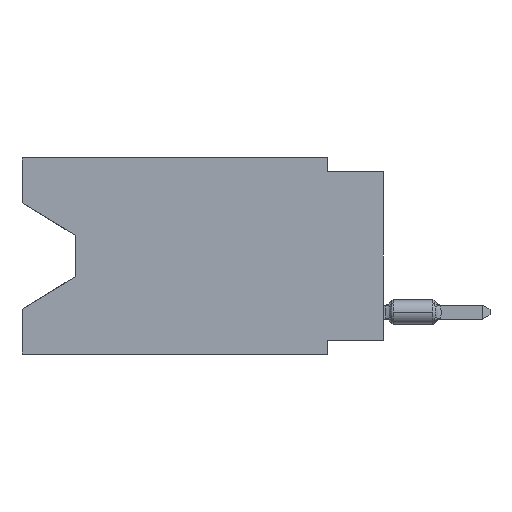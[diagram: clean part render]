
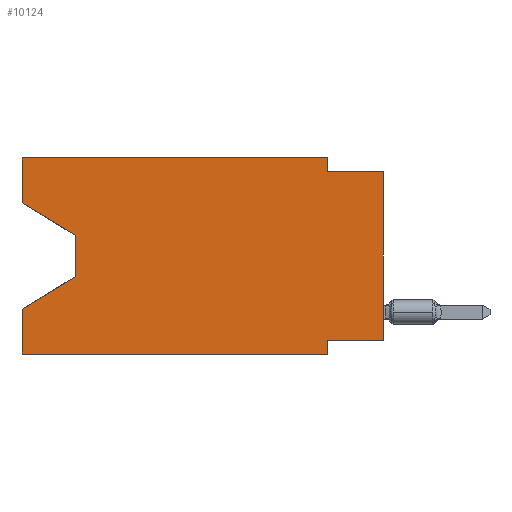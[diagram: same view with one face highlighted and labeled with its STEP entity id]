
A CAD part, left-side view. The second image highlights one B-rep face of the part: STEP entity #10124.
In plain terms, the highlighted planar face has unit normal (-1, 0, 0).
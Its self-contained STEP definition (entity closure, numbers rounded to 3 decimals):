
#159 = CARTESIAN_POINT ( 'NONE',  ( 0., 16.383, 0. ) ) ;
#282 = DIRECTION ( 'NONE',  ( 0., -0.855, -0.519 ) ) ;
#310 = VERTEX_POINT ( 'NONE', #6698 ) ;
#500 = CARTESIAN_POINT ( 'NONE',  ( 0., 2.54, -0.635 ) ) ;
#586 = ORIENTED_EDGE ( 'NONE', *, *, #6558, .F. ) ;
#632 = FACE_OUTER_BOUND ( 'NONE', #5957, .T. ) ;
#927 = VERTEX_POINT ( 'NONE', #4889 ) ;
#947 = LINE ( 'NONE', #3052, #4739 ) ;
#1186 = DIRECTION ( 'NONE',  ( 0., 0., -1. ) ) ;
#1225 = LINE ( 'NONE', #3193, #10870 ) ;
#1258 = VERTEX_POINT ( 'NONE', #9749 ) ;
#1430 = VERTEX_POINT ( 'NONE', #13397 ) ;
#1559 = ORIENTED_EDGE ( 'NONE', *, *, #10036, .F. ) ;
#1569 = VECTOR ( 'NONE', #1867, 1000. ) ;
#1867 = DIRECTION ( 'NONE',  ( 0., 0., 1. ) ) ;
#1986 = CARTESIAN_POINT ( 'NONE',  ( 0., 0., -0.635 ) ) ;
#2280 = CARTESIAN_POINT ( 'NONE',  ( 0., 13.97, -5.385 ) ) ;
#2596 = LINE ( 'NONE', #12904, #9210 ) ;
#2747 = VECTOR ( 'NONE', #8616, 1000. ) ;
#2762 = EDGE_CURVE ( 'NONE', #1430, #9212, #2888, .T. ) ;
#2861 = VECTOR ( 'NONE', #11768, 1000. ) ;
#2888 = LINE ( 'NONE', #12171, #1569 ) ;
#2956 = ORIENTED_EDGE ( 'NONE', *, *, #2762, .T. ) ;
#2991 = DIRECTION ( 'NONE',  ( 0., 0., -1. ) ) ;
#3017 = ORIENTED_EDGE ( 'NONE', *, *, #4580, .F. ) ;
#3052 = CARTESIAN_POINT ( 'NONE',  ( 0., 13.97, -5.385 ) ) ;
#3114 = VECTOR ( 'NONE', #8752, 1000. ) ;
#3193 = CARTESIAN_POINT ( 'NONE',  ( 0., 0., -8.255 ) ) ;
#3196 = ORIENTED_EDGE ( 'NONE', *, *, #9246, .T. ) ;
#3218 = VECTOR ( 'NONE', #2991, 1000. ) ;
#3431 = ORIENTED_EDGE ( 'NONE', *, *, #3661, .T. ) ;
#3661 = EDGE_CURVE ( 'NONE', #7202, #927, #12810, .T. ) ;
#3840 = CARTESIAN_POINT ( 'NONE',  ( 0., 16.383, 0. ) ) ;
#3955 = CARTESIAN_POINT ( 'NONE',  ( 0., 0., -0.635 ) ) ;
#3985 = AXIS2_PLACEMENT_3D ( 'NONE', #7921, #5612, #5863 ) ;
#4011 = VERTEX_POINT ( 'NONE', #2280 ) ;
#4580 = EDGE_CURVE ( 'NONE', #7357, #1258, #2596, .T. ) ;
#4739 = VECTOR ( 'NONE', #13354, 1000. ) ;
#4778 = LINE ( 'NONE', #8952, #3114 ) ;
#4889 = CARTESIAN_POINT ( 'NONE',  ( 0., 2.54, -8.89 ) ) ;
#4983 = LINE ( 'NONE', #9699, #12924 ) ;
#5260 = LINE ( 'NONE', #159, #2747 ) ;
#5420 = CARTESIAN_POINT ( 'NONE',  ( 0., 16.383, -6.852 ) ) ;
#5612 = DIRECTION ( 'NONE',  ( 1., 0., 0. ) ) ;
#5650 = LINE ( 'NONE', #10296, #3218 ) ;
#5844 = VERTEX_POINT ( 'NONE', #9049 ) ;
#5863 = DIRECTION ( 'NONE',  ( 0., 0., -1. ) ) ;
#5957 = EDGE_LOOP ( 'NONE', ( #3196, #12633, #12354, #12516, #3431, #586, #8407, #2956, #12439, #9367, #3017, #1559 ) ) ;
#6280 = EDGE_CURVE ( 'NONE', #1258, #9047, #8902, .T. ) ;
#6438 = EDGE_CURVE ( 'NONE', #7202, #7292, #5260, .T. ) ;
#6558 = EDGE_CURVE ( 'NONE', #5844, #927, #10531, .T. ) ;
#6698 = CARTESIAN_POINT ( 'NONE',  ( 0., 16.383, -2.038 ) ) ;
#6850 = CARTESIAN_POINT ( 'NONE',  ( 0., 13.97, -3.505 ) ) ;
#6876 = VECTOR ( 'NONE', #1186, 1000. ) ;
#7202 = VERTEX_POINT ( 'NONE', #8149 ) ;
#7292 = VERTEX_POINT ( 'NONE', #5420 ) ;
#7357 = VERTEX_POINT ( 'NONE', #3840 ) ;
#7617 = CARTESIAN_POINT ( 'NONE',  ( 0., 16.383, -8.89 ) ) ;
#7863 = CARTESIAN_POINT ( 'NONE',  ( 0., 2.54, 0. ) ) ;
#7921 = CARTESIAN_POINT ( 'NONE',  ( 0., 16.383, 0. ) ) ;
#7928 = EDGE_CURVE ( 'NONE', #9047, #9212, #13369, .T. ) ;
#8149 = CARTESIAN_POINT ( 'NONE',  ( 0., 16.383, -8.89 ) ) ;
#8306 = EDGE_CURVE ( 'NONE', #10998, #4011, #5650, .T. ) ;
#8323 = EDGE_CURVE ( 'NONE', #4011, #7292, #947, .T. ) ;
#8407 = ORIENTED_EDGE ( 'NONE', *, *, #8582, .F. ) ;
#8582 = EDGE_CURVE ( 'NONE', #1430, #5844, #1225, .T. ) ;
#8616 = DIRECTION ( 'NONE',  ( 0., 0., 1. ) ) ;
#8752 = DIRECTION ( 'NONE',  ( 0., 0., 1. ) ) ;
#8823 = PLANE ( 'NONE',  #3985 ) ;
#8902 = LINE ( 'NONE', #7863, #9721 ) ;
#8952 = CARTESIAN_POINT ( 'NONE',  ( 0., 16.383, 0. ) ) ;
#9047 = VERTEX_POINT ( 'NONE', #500 ) ;
#9049 = CARTESIAN_POINT ( 'NONE',  ( 0., 2.54, -8.255 ) ) ;
#9210 = VECTOR ( 'NONE', #9966, 1000. ) ;
#9212 = VERTEX_POINT ( 'NONE', #1986 ) ;
#9246 = EDGE_CURVE ( 'NONE', #310, #10998, #4983, .T. ) ;
#9367 = ORIENTED_EDGE ( 'NONE', *, *, #6280, .F. ) ;
#9473 = DIRECTION ( 'NONE',  ( 0., 1., 0. ) ) ;
#9699 = CARTESIAN_POINT ( 'NONE',  ( 0., 16.383, -2.038 ) ) ;
#9721 = VECTOR ( 'NONE', #11213, 1000. ) ;
#9749 = CARTESIAN_POINT ( 'NONE',  ( 0., 2.54, 0. ) ) ;
#9966 = DIRECTION ( 'NONE',  ( 0., -1., 0. ) ) ;
#10036 = EDGE_CURVE ( 'NONE', #310, #7357, #4778, .T. ) ;
#10124 = ADVANCED_FACE ( 'NONE', ( #632 ), #8823, .F. ) ;
#10296 = CARTESIAN_POINT ( 'NONE',  ( 0., 13.97, -3.505 ) ) ;
#10531 = LINE ( 'NONE', #11542, #6876 ) ;
#10634 = VECTOR ( 'NONE', #11129, 1000. ) ;
#10870 = VECTOR ( 'NONE', #9473, 1000. ) ;
#10998 = VERTEX_POINT ( 'NONE', #6850 ) ;
#11129 = DIRECTION ( 'NONE',  ( 0., -1., 0. ) ) ;
#11213 = DIRECTION ( 'NONE',  ( 0., 0., -1. ) ) ;
#11542 = CARTESIAN_POINT ( 'NONE',  ( 0., 2.54, -8.89 ) ) ;
#11768 = DIRECTION ( 'NONE',  ( 0., -1., 0. ) ) ;
#12171 = CARTESIAN_POINT ( 'NONE',  ( 0., 0., 0. ) ) ;
#12354 = ORIENTED_EDGE ( 'NONE', *, *, #8323, .T. ) ;
#12439 = ORIENTED_EDGE ( 'NONE', *, *, #7928, .F. ) ;
#12516 = ORIENTED_EDGE ( 'NONE', *, *, #6438, .F. ) ;
#12633 = ORIENTED_EDGE ( 'NONE', *, *, #8306, .T. ) ;
#12810 = LINE ( 'NONE', #7617, #2861 ) ;
#12904 = CARTESIAN_POINT ( 'NONE',  ( 0., 16.383, 0. ) ) ;
#12924 = VECTOR ( 'NONE', #282, 1000. ) ;
#13354 = DIRECTION ( 'NONE',  ( 0., 0.855, -0.519 ) ) ;
#13369 = LINE ( 'NONE', #3955, #10634 ) ;
#13397 = CARTESIAN_POINT ( 'NONE',  ( 0., 0., -8.255 ) ) ;
